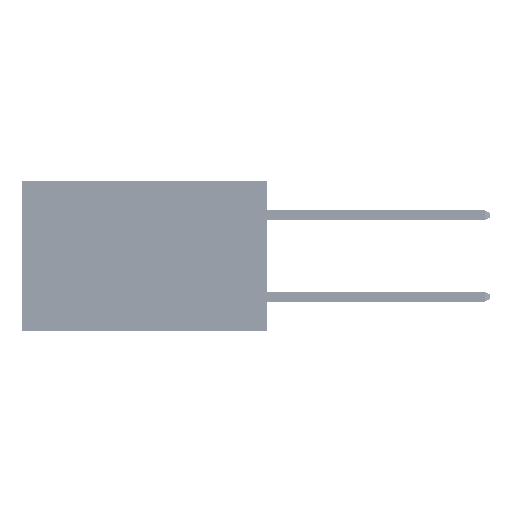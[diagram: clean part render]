
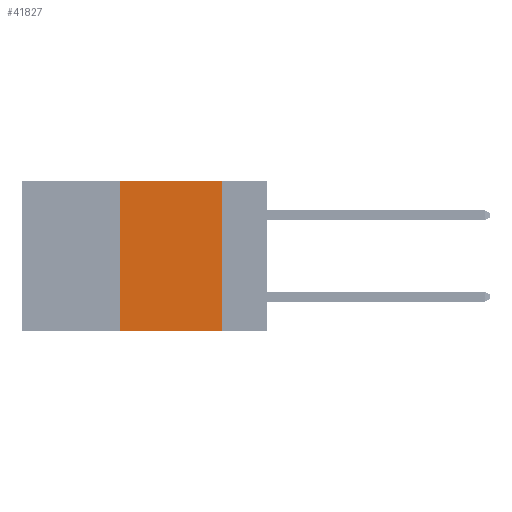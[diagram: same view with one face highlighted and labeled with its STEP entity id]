
A CAD part, left-side view. The second image highlights one B-rep face of the part: STEP entity #41827.
In plain terms, the highlighted planar face has unit normal (-1, 0, 0).
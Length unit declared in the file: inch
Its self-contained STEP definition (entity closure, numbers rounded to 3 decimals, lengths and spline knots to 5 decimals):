
#995 = CARTESIAN_POINT ( 'NONE',  ( 0., 0.11, 0. ) ) ;
#1013 = LINE ( 'NONE', #24952, #38322 ) ;
#2765 = AXIS2_PLACEMENT_3D ( 'NONE', #45198, #5562, #9036 ) ;
#3296 = DIRECTION ( 'NONE',  ( 0., -1., 0. ) ) ;
#3705 = DIRECTION ( 'NONE',  ( 0., 0., 1. ) ) ;
#4018 = LINE ( 'NONE', #29488, #24389 ) ;
#5562 = DIRECTION ( 'NONE',  ( 1., 0., 0. ) ) ;
#6266 = CARTESIAN_POINT ( 'NONE',  ( 0., 0.11, -0.37 ) ) ;
#9036 = DIRECTION ( 'NONE',  ( 0., 0., -1. ) ) ;
#9103 = ORIENTED_EDGE ( 'NONE', *, *, #16732, .T. ) ;
#11684 = CARTESIAN_POINT ( 'NONE',  ( 0., 0.36, 0. ) ) ;
#14875 = ORIENTED_EDGE ( 'NONE', *, *, #37527, .F. ) ;
#15973 = DIRECTION ( 'NONE',  ( 0., 0., -1. ) ) ;
#16732 = EDGE_CURVE ( 'NONE', #20015, #41063, #1013, .T. ) ;
#16906 = FACE_OUTER_BOUND ( 'NONE', #44317, .T. ) ;
#19773 = PLANE ( 'NONE',  #2765 ) ;
#20015 = VERTEX_POINT ( 'NONE', #39502 ) ;
#20249 = VERTEX_POINT ( 'NONE', #11684 ) ;
#21546 = CARTESIAN_POINT ( 'NONE',  ( 0., 0.11, 0. ) ) ;
#24389 = VECTOR ( 'NONE', #3705, 39.37008 ) ;
#24952 = CARTESIAN_POINT ( 'NONE',  ( 0., 0.6, -0.37 ) ) ;
#25256 = ORIENTED_EDGE ( 'NONE', *, *, #41691, .F. ) ;
#26948 = VECTOR ( 'NONE', #42857, 39.37008 ) ;
#29169 = LINE ( 'NONE', #39263, #26948 ) ;
#29488 = CARTESIAN_POINT ( 'NONE',  ( 0., 0.36, 0. ) ) ;
#31622 = EDGE_CURVE ( 'NONE', #20015, #20249, #4018, .T. ) ;
#31758 = ORIENTED_EDGE ( 'NONE', *, *, #31622, .F. ) ;
#32156 = VERTEX_POINT ( 'NONE', #21546 ) ;
#36714 = VECTOR ( 'NONE', #15973, 39.37008 ) ;
#37527 = EDGE_CURVE ( 'NONE', #20249, #32156, #29169, .T. ) ;
#38322 = VECTOR ( 'NONE', #3296, 39.37008 ) ;
#39263 = CARTESIAN_POINT ( 'NONE',  ( 0., 0.6, 0. ) ) ;
#39502 = CARTESIAN_POINT ( 'NONE',  ( 0., 0.36, -0.37 ) ) ;
#41063 = VERTEX_POINT ( 'NONE', #6266 ) ;
#41691 = EDGE_CURVE ( 'NONE', #32156, #41063, #45200, .T. ) ;
#41827 = ADVANCED_FACE ( 'NONE', ( #16906 ), #19773, .F. ) ;
#42857 = DIRECTION ( 'NONE',  ( 0., -1., 0. ) ) ;
#44317 = EDGE_LOOP ( 'NONE', ( #25256, #14875, #31758, #9103 ) ) ;
#45198 = CARTESIAN_POINT ( 'NONE',  ( 0., 0.6, 0. ) ) ;
#45200 = LINE ( 'NONE', #995, #36714 ) ;
